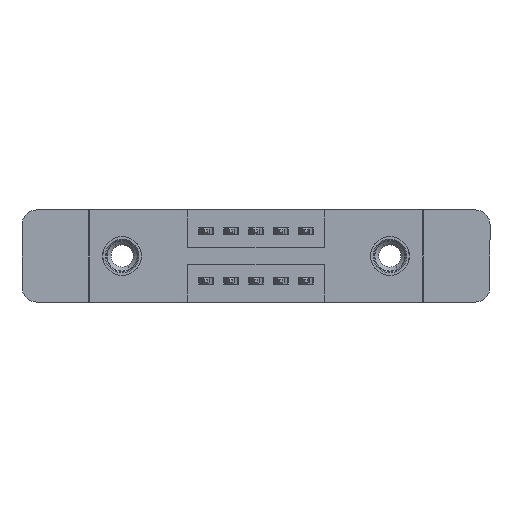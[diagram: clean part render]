
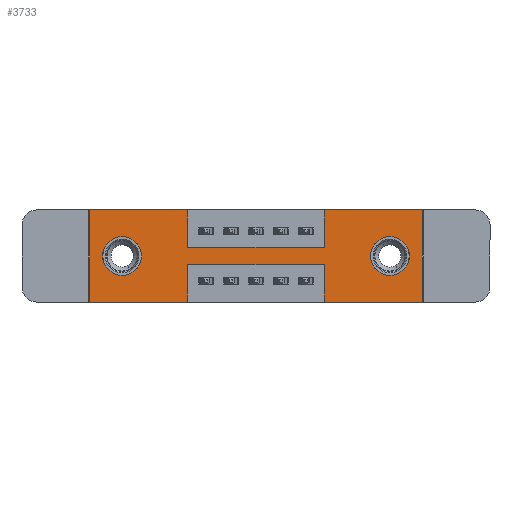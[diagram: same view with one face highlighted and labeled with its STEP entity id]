
A CAD part, front view. The second image highlights one B-rep face of the part: STEP entity #3733.
In plain terms, the highlighted planar face has unit normal (0, -1, 0).
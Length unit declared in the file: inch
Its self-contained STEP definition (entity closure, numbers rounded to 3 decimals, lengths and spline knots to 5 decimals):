
#179 = ORIENTED_EDGE ( 'NONE', *, *, #9519, .F. ) ;
#335 = CARTESIAN_POINT ( 'NONE',  ( 1.335, 0., 0. ) ) ;
#462 = CARTESIAN_POINT ( 'NONE',  ( 1.205, 0., -0.263 ) ) ;
#525 = EDGE_CURVE ( 'NONE', #1868, #10534, #925, .T. ) ;
#698 = DIRECTION ( 'NONE',  ( 0., 0., 1. ) ) ;
#925 = LINE ( 'NONE', #1035, #11794 ) ;
#994 = EDGE_CURVE ( 'NONE', #10664, #11908, #3528, .T. ) ;
#1035 = CARTESIAN_POINT ( 'NONE',  ( 0.3925, 0., 0. ) ) ;
#1234 = DIRECTION ( 'NONE',  ( 0., 0., -1. ) ) ;
#1268 = CARTESIAN_POINT ( 'NONE',  ( 0.9425, 0., -0.15 ) ) ;
#1292 = AXIS2_PLACEMENT_3D ( 'NONE', #9575, #3108, #10656 ) ;
#1407 = DIRECTION ( 'NONE',  ( 0., 0., -1. ) ) ;
#1411 = DIRECTION ( 'NONE',  ( 0., -1., 0. ) ) ;
#1419 = CARTESIAN_POINT ( 'NONE',  ( 0., 0., -0.37 ) ) ;
#1440 = PLANE ( 'NONE',  #5286 ) ;
#1444 = CARTESIAN_POINT ( 'NONE',  ( 0., 0., -0.37 ) ) ;
#1488 = DIRECTION ( 'NONE',  ( 0., 0., 1. ) ) ;
#1719 = CARTESIAN_POINT ( 'NONE',  ( 0.3925, 0., -0.22 ) ) ;
#1868 = VERTEX_POINT ( 'NONE', #8931 ) ;
#2018 = CARTESIAN_POINT ( 'NONE',  ( 1.205, 0., -0.107 ) ) ;
#2070 = DIRECTION ( 'NONE',  ( 0., 0., -1. ) ) ;
#2120 = CARTESIAN_POINT ( 'NONE',  ( 0.3925, 0., -0.37 ) ) ;
#2327 = VERTEX_POINT ( 'NONE', #13419 ) ;
#2373 = CARTESIAN_POINT ( 'NONE',  ( 0.3925, 0., -0.15 ) ) ;
#2391 = VERTEX_POINT ( 'NONE', #12984 ) ;
#2452 = LINE ( 'NONE', #4716, #11750 ) ;
#2536 = DIRECTION ( 'NONE',  ( 0., 0., 1. ) ) ;
#2663 = LINE ( 'NONE', #1419, #8121 ) ;
#2779 = ORIENTED_EDGE ( 'NONE', *, *, #8027, .F. ) ;
#2786 = EDGE_CURVE ( 'NONE', #11908, #1868, #10063, .T. ) ;
#2932 = VERTEX_POINT ( 'NONE', #8902 ) ;
#3108 = DIRECTION ( 'NONE',  ( 0., 1., 0. ) ) ;
#3121 = DIRECTION ( 'NONE',  ( 1., 0., 0. ) ) ;
#3305 = CARTESIAN_POINT ( 'NONE',  ( 0., 0., 0. ) ) ;
#3352 = DIRECTION ( 'NONE',  ( 1., 0., 0. ) ) ;
#3460 = CARTESIAN_POINT ( 'NONE',  ( 0.3925, 0., -0.15 ) ) ;
#3464 = LINE ( 'NONE', #2120, #11382 ) ;
#3528 = LINE ( 'NONE', #6409, #11780 ) ;
#3598 = EDGE_CURVE ( 'NONE', #10534, #4790, #6348, .T. ) ;
#3631 = EDGE_CURVE ( 'NONE', #9326, #4942, #3464, .T. ) ;
#3641 = VERTEX_POINT ( 'NONE', #2018 ) ;
#3733 = ADVANCED_FACE ( 'NONE', ( #6339, #3797, #9187 ), #1440, .T. ) ;
#3794 = CARTESIAN_POINT ( 'NONE',  ( 0.3925, 0., -0.37 ) ) ;
#3797 = FACE_BOUND ( 'NONE', #7350, .T. ) ;
#3870 = DIRECTION ( 'NONE',  ( 0., 1., 0. ) ) ;
#3895 = VERTEX_POINT ( 'NONE', #335 ) ;
#4176 = VECTOR ( 'NONE', #7494, 39.37008 ) ;
#4232 = ORIENTED_EDGE ( 'NONE', *, *, #9229, .F. ) ;
#4266 = ORIENTED_EDGE ( 'NONE', *, *, #12450, .T. ) ;
#4306 = ORIENTED_EDGE ( 'NONE', *, *, #12966, .T. ) ;
#4345 = VECTOR ( 'NONE', #9993, 39.37008 ) ;
#4366 = DIRECTION ( 'NONE',  ( 0., 1., 0. ) ) ;
#4370 = CIRCLE ( 'NONE', #6332, 0.078 ) ;
#4427 = ORIENTED_EDGE ( 'NONE', *, *, #13851, .F. ) ;
#4619 = ORIENTED_EDGE ( 'NONE', *, *, #3598, .F. ) ;
#4644 = EDGE_LOOP ( 'NONE', ( #4266, #5312 ) ) ;
#4716 = CARTESIAN_POINT ( 'NONE',  ( 1.335, 0., 0. ) ) ;
#4790 = VERTEX_POINT ( 'NONE', #1268 ) ;
#4894 = CARTESIAN_POINT ( 'NONE',  ( 0., 0., -0.37 ) ) ;
#4942 = VERTEX_POINT ( 'NONE', #3794 ) ;
#5129 = ORIENTED_EDGE ( 'NONE', *, *, #8795, .T. ) ;
#5286 = AXIS2_PLACEMENT_3D ( 'NONE', #1444, #1411, #1407 ) ;
#5302 = CARTESIAN_POINT ( 'NONE',  ( 0.9425, 0., -0.37 ) ) ;
#5312 = ORIENTED_EDGE ( 'NONE', *, *, #10861, .T. ) ;
#5425 = ORIENTED_EDGE ( 'NONE', *, *, #525, .F. ) ;
#5755 = ORIENTED_EDGE ( 'NONE', *, *, #2786, .F. ) ;
#5966 = DIRECTION ( 'NONE',  ( -1., 0., 0. ) ) ;
#6099 = EDGE_CURVE ( 'NONE', #7920, #8968, #7486, .T. ) ;
#6260 = DIRECTION ( 'NONE',  ( -1., 0., 0. ) ) ;
#6332 = AXIS2_PLACEMENT_3D ( 'NONE', #10312, #3870, #11399 ) ;
#6339 = FACE_BOUND ( 'NONE', #4644, .T. ) ;
#6348 = LINE ( 'NONE', #2373, #12389 ) ;
#6409 = CARTESIAN_POINT ( 'NONE',  ( 0., 0., 0. ) ) ;
#6536 = CIRCLE ( 'NONE', #10200, 0.078 ) ;
#7001 = ORIENTED_EDGE ( 'NONE', *, *, #8050, .F. ) ;
#7054 = LINE ( 'NONE', #5302, #4176 ) ;
#7192 = ORIENTED_EDGE ( 'NONE', *, *, #994, .F. ) ;
#7272 = DIRECTION ( 'NONE',  ( 0., 1., 0. ) ) ;
#7350 = EDGE_LOOP ( 'NONE', ( #5129, #4306 ) ) ;
#7390 = ORIENTED_EDGE ( 'NONE', *, *, #10317, .F. ) ;
#7486 = LINE ( 'NONE', #4894, #12836 ) ;
#7494 = DIRECTION ( 'NONE',  ( 0., 0., 1. ) ) ;
#7920 = VERTEX_POINT ( 'NONE', #12069 ) ;
#7965 = CARTESIAN_POINT ( 'NONE',  ( 0.9425, 0., 0. ) ) ;
#8003 = CIRCLE ( 'NONE', #9767, 0.078 ) ;
#8027 = EDGE_CURVE ( 'NONE', #4790, #2391, #10106, .T. ) ;
#8050 = EDGE_CURVE ( 'NONE', #4942, #10664, #2663, .T. ) ;
#8121 = VECTOR ( 'NONE', #9074, 39.37008 ) ;
#8255 = ORIENTED_EDGE ( 'NONE', *, *, #3631, .F. ) ;
#8454 = CARTESIAN_POINT ( 'NONE',  ( 0., 0., 0. ) ) ;
#8456 = VECTOR ( 'NONE', #2536, 39.37008 ) ;
#8550 = CARTESIAN_POINT ( 'NONE',  ( 0.9425, 0., -0.37 ) ) ;
#8631 = EDGE_LOOP ( 'NONE', ( #8255, #7390, #179, #11453, #4232, #4427, #2779, #4619, #5425, #5755, #7192, #7001 ) ) ;
#8795 = EDGE_CURVE ( 'NONE', #9421, #2327, #4370, .T. ) ;
#8902 = CARTESIAN_POINT ( 'NONE',  ( 0.9425, 0., -0.22 ) ) ;
#8931 = CARTESIAN_POINT ( 'NONE',  ( 0.3925, 0., 0. ) ) ;
#8968 = VERTEX_POINT ( 'NONE', #8550 ) ;
#8970 = VECTOR ( 'NONE', #3352, 39.37008 ) ;
#9038 = VECTOR ( 'NONE', #6260, 39.37008 ) ;
#9040 = DIRECTION ( 'NONE',  ( 0., 0., -1. ) ) ;
#9074 = DIRECTION ( 'NONE',  ( -1., 0., 0. ) ) ;
#9187 = FACE_OUTER_BOUND ( 'NONE', #8631, .T. ) ;
#9229 = EDGE_CURVE ( 'NONE', #3895, #7920, #2452, .T. ) ;
#9326 = VERTEX_POINT ( 'NONE', #1719 ) ;
#9421 = VERTEX_POINT ( 'NONE', #11613 ) ;
#9457 = CARTESIAN_POINT ( 'NONE',  ( 0.3925, 0., -0.22 ) ) ;
#9519 = EDGE_CURVE ( 'NONE', #8968, #2932, #7054, .T. ) ;
#9575 = CARTESIAN_POINT ( 'NONE',  ( 1.205, 0., -0.185 ) ) ;
#9767 = AXIS2_PLACEMENT_3D ( 'NONE', #13691, #7272, #698 ) ;
#9962 = CARTESIAN_POINT ( 'NONE',  ( 0., 0., 0. ) ) ;
#9993 = DIRECTION ( 'NONE',  ( 1., 0., 0. ) ) ;
#10063 = LINE ( 'NONE', #9962, #4345 ) ;
#10106 = LINE ( 'NONE', #7965, #8456 ) ;
#10200 = AXIS2_PLACEMENT_3D ( 'NONE', #10805, #4366, #11874 ) ;
#10240 = CARTESIAN_POINT ( 'NONE',  ( 0., 0., -0.37 ) ) ;
#10312 = CARTESIAN_POINT ( 'NONE',  ( 0.13, 0., -0.185 ) ) ;
#10317 = EDGE_CURVE ( 'NONE', #2932, #9326, #11886, .T. ) ;
#10534 = VERTEX_POINT ( 'NONE', #3460 ) ;
#10656 = DIRECTION ( 'NONE',  ( 0., 0., -1. ) ) ;
#10664 = VERTEX_POINT ( 'NONE', #10240 ) ;
#10805 = CARTESIAN_POINT ( 'NONE',  ( 1.205, 0., -0.185 ) ) ;
#10852 = CIRCLE ( 'NONE', #1292, 0.078 ) ;
#10861 = EDGE_CURVE ( 'NONE', #14078, #3641, #6536, .T. ) ;
#11382 = VECTOR ( 'NONE', #2070, 39.37008 ) ;
#11399 = DIRECTION ( 'NONE',  ( 0., 0., 1. ) ) ;
#11453 = ORIENTED_EDGE ( 'NONE', *, *, #6099, .F. ) ;
#11613 = CARTESIAN_POINT ( 'NONE',  ( 0.13, 0., -0.107 ) ) ;
#11750 = VECTOR ( 'NONE', #9040, 39.37008 ) ;
#11780 = VECTOR ( 'NONE', #1488, 39.37008 ) ;
#11794 = VECTOR ( 'NONE', #1234, 39.37008 ) ;
#11812 = LINE ( 'NONE', #3305, #8970 ) ;
#11874 = DIRECTION ( 'NONE',  ( 0., 0., -1. ) ) ;
#11886 = LINE ( 'NONE', #9457, #9038 ) ;
#11908 = VERTEX_POINT ( 'NONE', #8454 ) ;
#12069 = CARTESIAN_POINT ( 'NONE',  ( 1.335, 0., -0.37 ) ) ;
#12389 = VECTOR ( 'NONE', #3121, 39.37008 ) ;
#12450 = EDGE_CURVE ( 'NONE', #3641, #14078, #10852, .T. ) ;
#12836 = VECTOR ( 'NONE', #5966, 39.37008 ) ;
#12966 = EDGE_CURVE ( 'NONE', #2327, #9421, #8003, .T. ) ;
#12984 = CARTESIAN_POINT ( 'NONE',  ( 0.9425, 0., 0. ) ) ;
#13419 = CARTESIAN_POINT ( 'NONE',  ( 0.13, 0., -0.263 ) ) ;
#13691 = CARTESIAN_POINT ( 'NONE',  ( 0.13, 0., -0.185 ) ) ;
#13851 = EDGE_CURVE ( 'NONE', #2391, #3895, #11812, .T. ) ;
#14078 = VERTEX_POINT ( 'NONE', #462 ) ;
